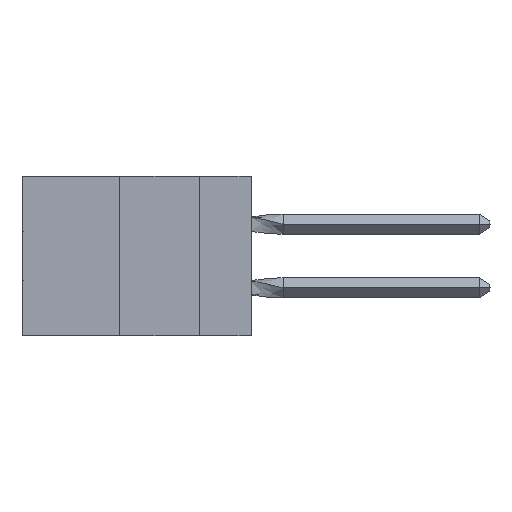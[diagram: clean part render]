
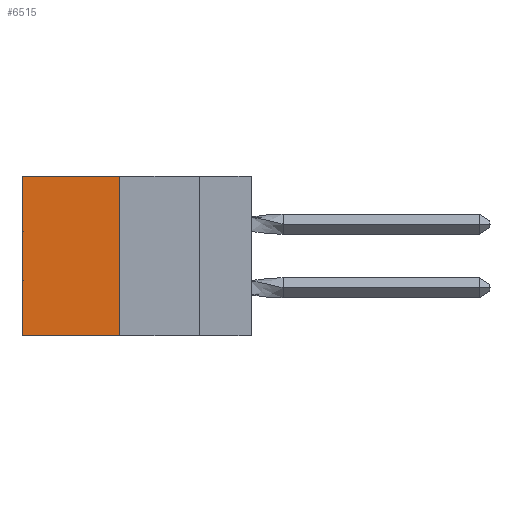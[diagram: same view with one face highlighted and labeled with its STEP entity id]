
A CAD part, left-side view. The second image highlights one B-rep face of the part: STEP entity #6515.
In plain terms, the highlighted planar face has unit normal (-1, 0, 0).
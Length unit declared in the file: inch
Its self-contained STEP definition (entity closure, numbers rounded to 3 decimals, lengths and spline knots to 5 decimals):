
#1099 = VECTOR ( 'NONE', #40736, 39.37008 ) ;
#1155 = EDGE_CURVE ( 'NONE', #40117, #18202, #3156, .T. ) ;
#1544 = EDGE_CURVE ( 'NONE', #40117, #7252, #34690, .T. ) ;
#3156 = LINE ( 'NONE', #26321, #1099 ) ;
#3309 = VERTEX_POINT ( 'NONE', #28958 ) ;
#3721 = LINE ( 'NONE', #22862, #25956 ) ;
#5388 = LINE ( 'NONE', #15473, #26097 ) ;
#5528 = CARTESIAN_POINT ( 'NONE',  ( 0.305, 0.413, 0. ) ) ;
#6515 = ADVANCED_FACE ( 'NONE', ( #8892 ), #17218, .F. ) ;
#7252 = VERTEX_POINT ( 'NONE', #33215 ) ;
#7335 = EDGE_LOOP ( 'NONE', ( #36818, #9451, #17415, #35867 ) ) ;
#8892 = FACE_OUTER_BOUND ( 'NONE', #7335, .T. ) ;
#9451 = ORIENTED_EDGE ( 'NONE', *, *, #37492, .F. ) ;
#12127 = DIRECTION ( 'NONE',  ( 0., 1., 0. ) ) ;
#12186 = CARTESIAN_POINT ( 'NONE',  ( 0.305, 0.413, -0.5 ) ) ;
#12581 = DIRECTION ( 'NONE',  ( 0., 1., 0. ) ) ;
#13030 = DIRECTION ( 'NONE',  ( 0., 0., -1. ) ) ;
#15473 = CARTESIAN_POINT ( 'NONE',  ( 0.305, 0.413, -0.5 ) ) ;
#17218 = PLANE ( 'NONE',  #40385 ) ;
#17415 = ORIENTED_EDGE ( 'NONE', *, *, #1155, .F. ) ;
#18202 = VERTEX_POINT ( 'NONE', #12186 ) ;
#20930 = EDGE_CURVE ( 'NONE', #7252, #3309, #3721, .T. ) ;
#22862 = CARTESIAN_POINT ( 'NONE',  ( 0.305, 0.72, -0.5 ) ) ;
#24389 = VECTOR ( 'NONE', #12581, 39.37008 ) ;
#25956 = VECTOR ( 'NONE', #13030, 39.37008 ) ;
#26097 = VECTOR ( 'NONE', #12127, 39.37008 ) ;
#26321 = CARTESIAN_POINT ( 'NONE',  ( 0.305, 0.413, -0.5 ) ) ;
#28958 = CARTESIAN_POINT ( 'NONE',  ( 0.305, 0.72, -0.5 ) ) ;
#30457 = CARTESIAN_POINT ( 'NONE',  ( 0.305, 0.413, -0.5 ) ) ;
#30739 = DIRECTION ( 'NONE',  ( 0., 0., -1. ) ) ;
#33215 = CARTESIAN_POINT ( 'NONE',  ( 0.305, 0.72, 0. ) ) ;
#34690 = LINE ( 'NONE', #42100, #24389 ) ;
#35867 = ORIENTED_EDGE ( 'NONE', *, *, #1544, .T. ) ;
#36818 = ORIENTED_EDGE ( 'NONE', *, *, #20930, .T. ) ;
#37090 = DIRECTION ( 'NONE',  ( 1., 0., 0. ) ) ;
#37492 = EDGE_CURVE ( 'NONE', #18202, #3309, #5388, .T. ) ;
#40117 = VERTEX_POINT ( 'NONE', #5528 ) ;
#40385 = AXIS2_PLACEMENT_3D ( 'NONE', #30457, #37090, #30739 ) ;
#40736 = DIRECTION ( 'NONE',  ( 0., 0., -1. ) ) ;
#42100 = CARTESIAN_POINT ( 'NONE',  ( 0.305, 0.413, 0. ) ) ;
